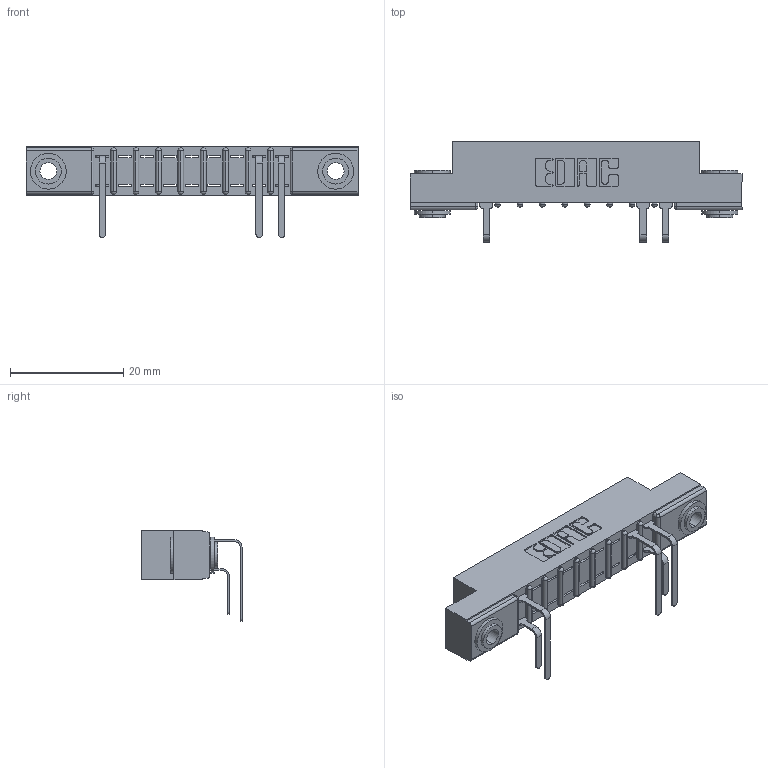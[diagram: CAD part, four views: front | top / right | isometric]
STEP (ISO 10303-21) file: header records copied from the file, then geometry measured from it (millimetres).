
FILE_DESCRIPTION (( 'STEP AP203' ), '1' );
FILE_NAME ('307-018-559-203.STEP', '2018-08-03T23:38:49', ( '' ), ( '' ), 'SwSTEP 2.0', 'SolidWorks 2016', '' );
FILE_SCHEMA (( 'CONFIG_CONTROL_DESIGN' ));
Length unit declared in the file: inch
Products named in the file (5): 345-250-002_345-250-002-102; 307-018-559-203; 307 Part_.156 Dia Mounting Holes; 307-290-001_558 559 - 1 (Single); 307-290-001_559 - 2 (Single)
Assembly tree (8 placements, depth 2):
  307-018-559-203
    307 Part_.156 Dia Mounting Holes
    307-290-001_558 559 - 1 (Single)  x2
    307-290-001_559 - 2 (Single)  x3
    345-250-002_345-250-002-102  x2
Bounding box: 58.67 x 17.69 x 16.08 mm (x, y, z)
Volume: 3696.2 mm3; surface area: 5238.4 mm2
Topology: 8 solids, 8 shells, 560 faces, 1561 edges, 1002 vertices
Faces by surface type: plane 337, cylinder 195, sphere 20, cone 8
Entity records: 14168 total; most frequent: CARTESIAN_POINT 2367, ORIENTED_EDGE 2346, DIRECTION 2333, EDGE_CURVE 1173, VECTOR 877, LINE 877, VERTEX_POINT 762, AXIS2_PLACEMENT_3D 728
